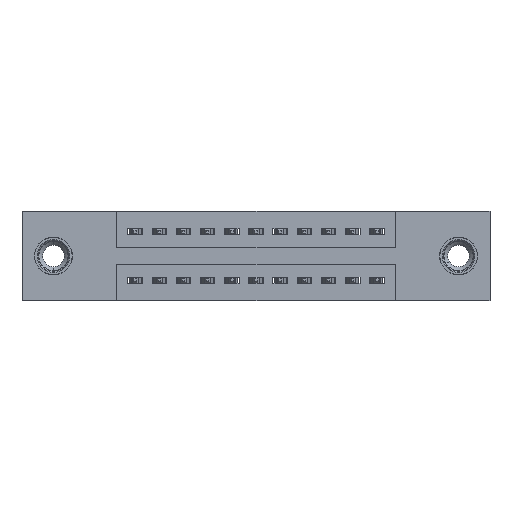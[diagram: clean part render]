
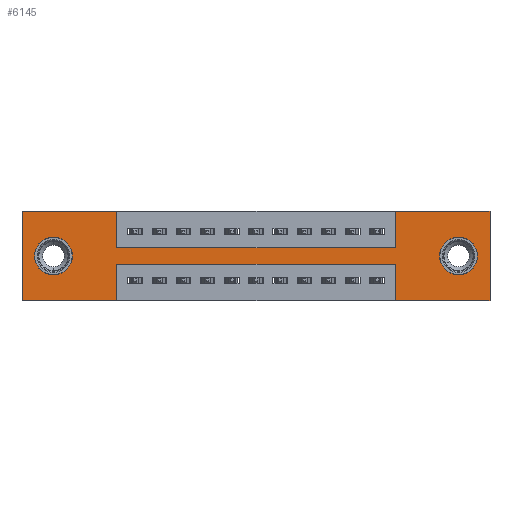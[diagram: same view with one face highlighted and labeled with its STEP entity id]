
A CAD part, front view. The second image highlights one B-rep face of the part: STEP entity #6145.
In plain terms, the highlighted planar face has unit normal (0, -1, 0).
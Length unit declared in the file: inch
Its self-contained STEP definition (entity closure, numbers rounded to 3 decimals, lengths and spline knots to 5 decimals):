
#20 = VERTEX_POINT ( 'NONE', #11122 ) ;
#23 = ORIENTED_EDGE ( 'NONE', *, *, #6052, .F. ) ;
#128 = ORIENTED_EDGE ( 'NONE', *, *, #2703, .F. ) ;
#165 = VERTEX_POINT ( 'NONE', #11045 ) ;
#206 = DIRECTION ( 'NONE',  ( 0., 0., 1. ) ) ;
#315 = EDGE_CURVE ( 'NONE', #11747, #10809, #11409, .T. ) ;
#462 = VECTOR ( 'NONE', #12750, 39.37008 ) ;
#887 = ORIENTED_EDGE ( 'NONE', *, *, #10371, .F. ) ;
#1019 = CARTESIAN_POINT ( 'NONE',  ( 1.935, 0., -0.37 ) ) ;
#1023 = VERTEX_POINT ( 'NONE', #4178 ) ;
#1107 = LINE ( 'NONE', #5156, #462 ) ;
#1495 = DIRECTION ( 'NONE',  ( -1., 0., 0. ) ) ;
#1529 = FACE_BOUND ( 'NONE', #7340, .T. ) ;
#1684 = VERTEX_POINT ( 'NONE', #13125 ) ;
#2119 = CARTESIAN_POINT ( 'NONE',  ( 0.3925, 0., -0.22 ) ) ;
#2204 = CARTESIAN_POINT ( 'NONE',  ( 0.13, 0., -0.185 ) ) ;
#2251 = CARTESIAN_POINT ( 'NONE',  ( 0.3925, 0., 0. ) ) ;
#2261 = LINE ( 'NONE', #10797, #5659 ) ;
#2303 = LINE ( 'NONE', #10645, #5187 ) ;
#2341 = AXIS2_PLACEMENT_3D ( 'NONE', #2204, #13065, #3444 ) ;
#2390 = VECTOR ( 'NONE', #1495, 39.37008 ) ;
#2434 = AXIS2_PLACEMENT_3D ( 'NONE', #13974, #2970, #11671 ) ;
#2435 = CARTESIAN_POINT ( 'NONE',  ( 0., 0., -0.37 ) ) ;
#2541 = EDGE_CURVE ( 'NONE', #13848, #13836, #4498, .T. ) ;
#2703 = EDGE_CURVE ( 'NONE', #4501, #13052, #9428, .T. ) ;
#2825 = CIRCLE ( 'NONE', #9827, 0.078 ) ;
#2970 = DIRECTION ( 'NONE',  ( 0., -1., 0. ) ) ;
#2999 = ORIENTED_EDGE ( 'NONE', *, *, #12667, .F. ) ;
#3106 = PLANE ( 'NONE',  #2434 ) ;
#3217 = VECTOR ( 'NONE', #10307, 39.37008 ) ;
#3347 = CARTESIAN_POINT ( 'NONE',  ( 0.13, 0., -0.107 ) ) ;
#3364 = CARTESIAN_POINT ( 'NONE',  ( 1.805, 0., -0.107 ) ) ;
#3444 = DIRECTION ( 'NONE',  ( 0., 0., 1. ) ) ;
#3503 = CARTESIAN_POINT ( 'NONE',  ( 0.3925, 0., -0.37 ) ) ;
#3883 = VECTOR ( 'NONE', #206, 39.37008 ) ;
#3990 = EDGE_CURVE ( 'NONE', #11073, #4501, #4802, .T. ) ;
#4178 = CARTESIAN_POINT ( 'NONE',  ( 1.935, 0., 0. ) ) ;
#4283 = VERTEX_POINT ( 'NONE', #6856 ) ;
#4307 = DIRECTION ( 'NONE',  ( 0., 1., 0. ) ) ;
#4315 = EDGE_CURVE ( 'NONE', #20, #11073, #8344, .T. ) ;
#4358 = CARTESIAN_POINT ( 'NONE',  ( 1.5425, 0., -0.37 ) ) ;
#4456 = VECTOR ( 'NONE', #9058, 39.37008 ) ;
#4498 = LINE ( 'NONE', #5763, #5514 ) ;
#4501 = VERTEX_POINT ( 'NONE', #6709 ) ;
#4526 = DIRECTION ( 'NONE',  ( 0., 0., -1. ) ) ;
#4534 = ORIENTED_EDGE ( 'NONE', *, *, #10204, .F. ) ;
#4769 = FACE_BOUND ( 'NONE', #14020, .T. ) ;
#4802 = LINE ( 'NONE', #2251, #5832 ) ;
#4848 = ORIENTED_EDGE ( 'NONE', *, *, #2541, .F. ) ;
#4930 = AXIS2_PLACEMENT_3D ( 'NONE', #10703, #9582, #11910 ) ;
#5156 = CARTESIAN_POINT ( 'NONE',  ( 1.935, 0., 0. ) ) ;
#5187 = VECTOR ( 'NONE', #11845, 39.37008 ) ;
#5188 = EDGE_CURVE ( 'NONE', #13836, #9325, #6814, .T. ) ;
#5395 = DIRECTION ( 'NONE',  ( -1., 0., 0. ) ) ;
#5418 = DIRECTION ( 'NONE',  ( 1., 0., 0. ) ) ;
#5426 = DIRECTION ( 'NONE',  ( 1., 0., 0. ) ) ;
#5514 = VECTOR ( 'NONE', #4526, 39.37008 ) ;
#5659 = VECTOR ( 'NONE', #5395, 39.37008 ) ;
#5763 = CARTESIAN_POINT ( 'NONE',  ( 0.3925, 0., -0.37 ) ) ;
#5832 = VECTOR ( 'NONE', #10734, 39.37008 ) ;
#5835 = ORIENTED_EDGE ( 'NONE', *, *, #8683, .F. ) ;
#5969 = ORIENTED_EDGE ( 'NONE', *, *, #11640, .F. ) ;
#6052 = EDGE_CURVE ( 'NONE', #8510, #1023, #6116, .T. ) ;
#6116 = LINE ( 'NONE', #9300, #3217 ) ;
#6145 = ADVANCED_FACE ( 'NONE', ( #4769, #1529, #9846 ), #3106, .T. ) ;
#6447 = CARTESIAN_POINT ( 'NONE',  ( 1.805, 0., -0.185 ) ) ;
#6582 = EDGE_CURVE ( 'NONE', #11406, #4283, #8632, .T. ) ;
#6709 = CARTESIAN_POINT ( 'NONE',  ( 0.3925, 0., -0.15 ) ) ;
#6809 = CARTESIAN_POINT ( 'NONE',  ( 0., 0., 0. ) ) ;
#6814 = LINE ( 'NONE', #2435, #12766 ) ;
#6856 = CARTESIAN_POINT ( 'NONE',  ( 0.13, 0., -0.263 ) ) ;
#6922 = DIRECTION ( 'NONE',  ( 0., 0., 1. ) ) ;
#6979 = CARTESIAN_POINT ( 'NONE',  ( 1.5425, 0., 0. ) ) ;
#7340 = EDGE_LOOP ( 'NONE', ( #11439, #11512 ) ) ;
#7367 = ORIENTED_EDGE ( 'NONE', *, *, #8702, .F. ) ;
#8245 = ORIENTED_EDGE ( 'NONE', *, *, #3990, .F. ) ;
#8321 = CARTESIAN_POINT ( 'NONE',  ( 0.3925, 0., -0.22 ) ) ;
#8344 = LINE ( 'NONE', #6809, #11421 ) ;
#8510 = VERTEX_POINT ( 'NONE', #6979 ) ;
#8632 = CIRCLE ( 'NONE', #10436, 0.078 ) ;
#8683 = EDGE_CURVE ( 'NONE', #1023, #13302, #1107, .T. ) ;
#8702 = EDGE_CURVE ( 'NONE', #9325, #20, #2303, .T. ) ;
#8724 = DIRECTION ( 'NONE',  ( 0., 0., -1. ) ) ;
#8741 = VECTOR ( 'NONE', #5418, 39.37008 ) ;
#8978 = CIRCLE ( 'NONE', #2341, 0.078 ) ;
#9058 = DIRECTION ( 'NONE',  ( 0., 0., 1. ) ) ;
#9300 = CARTESIAN_POINT ( 'NONE',  ( 0., 0., 0. ) ) ;
#9325 = VERTEX_POINT ( 'NONE', #10581 ) ;
#9428 = LINE ( 'NONE', #11932, #8741 ) ;
#9546 = LINE ( 'NONE', #11237, #4456 ) ;
#9582 = DIRECTION ( 'NONE',  ( 0., 1., 0. ) ) ;
#9827 = AXIS2_PLACEMENT_3D ( 'NONE', #6447, #4307, #8724 ) ;
#9846 = FACE_OUTER_BOUND ( 'NONE', #10379, .T. ) ;
#10076 = DIRECTION ( 'NONE',  ( -1., 0., 0. ) ) ;
#10204 = EDGE_CURVE ( 'NONE', #13302, #165, #2261, .T. ) ;
#10307 = DIRECTION ( 'NONE',  ( 1., 0., 0. ) ) ;
#10371 = EDGE_CURVE ( 'NONE', #13052, #8510, #9546, .T. ) ;
#10379 = EDGE_LOOP ( 'NONE', ( #4848, #5969, #2999, #4534, #5835, #23, #887, #128, #8245, #12338, #7367, #13858 ) ) ;
#10436 = AXIS2_PLACEMENT_3D ( 'NONE', #13606, #13417, #6922 ) ;
#10469 = CARTESIAN_POINT ( 'NONE',  ( 1.5425, 0., -0.15 ) ) ;
#10581 = CARTESIAN_POINT ( 'NONE',  ( 0., 0., -0.37 ) ) ;
#10645 = CARTESIAN_POINT ( 'NONE',  ( 0., 0., 0. ) ) ;
#10703 = CARTESIAN_POINT ( 'NONE',  ( 1.805, 0., -0.185 ) ) ;
#10734 = DIRECTION ( 'NONE',  ( 0., 0., -1. ) ) ;
#10797 = CARTESIAN_POINT ( 'NONE',  ( 0., 0., -0.37 ) ) ;
#10809 = VERTEX_POINT ( 'NONE', #3364 ) ;
#11045 = CARTESIAN_POINT ( 'NONE',  ( 1.5425, 0., -0.37 ) ) ;
#11073 = VERTEX_POINT ( 'NONE', #13703 ) ;
#11122 = CARTESIAN_POINT ( 'NONE',  ( 0., 0., 0. ) ) ;
#11237 = CARTESIAN_POINT ( 'NONE',  ( 1.5425, 0., 0. ) ) ;
#11406 = VERTEX_POINT ( 'NONE', #3347 ) ;
#11409 = CIRCLE ( 'NONE', #4930, 0.078 ) ;
#11421 = VECTOR ( 'NONE', #5426, 39.37008 ) ;
#11439 = ORIENTED_EDGE ( 'NONE', *, *, #6582, .T. ) ;
#11512 = ORIENTED_EDGE ( 'NONE', *, *, #13300, .T. ) ;
#11640 = EDGE_CURVE ( 'NONE', #1684, #13848, #13926, .T. ) ;
#11671 = DIRECTION ( 'NONE',  ( 0., 0., -1. ) ) ;
#11734 = ORIENTED_EDGE ( 'NONE', *, *, #13954, .T. ) ;
#11747 = VERTEX_POINT ( 'NONE', #12654 ) ;
#11845 = DIRECTION ( 'NONE',  ( 0., 0., 1. ) ) ;
#11910 = DIRECTION ( 'NONE',  ( 0., 0., -1. ) ) ;
#11932 = CARTESIAN_POINT ( 'NONE',  ( 0.3925, 0., -0.15 ) ) ;
#12222 = LINE ( 'NONE', #4358, #3883 ) ;
#12338 = ORIENTED_EDGE ( 'NONE', *, *, #4315, .F. ) ;
#12654 = CARTESIAN_POINT ( 'NONE',  ( 1.805, 0., -0.263 ) ) ;
#12667 = EDGE_CURVE ( 'NONE', #165, #1684, #12222, .T. ) ;
#12750 = DIRECTION ( 'NONE',  ( 0., 0., -1. ) ) ;
#12766 = VECTOR ( 'NONE', #10076, 39.37008 ) ;
#13016 = ORIENTED_EDGE ( 'NONE', *, *, #315, .T. ) ;
#13052 = VERTEX_POINT ( 'NONE', #10469 ) ;
#13065 = DIRECTION ( 'NONE',  ( 0., 1., 0. ) ) ;
#13125 = CARTESIAN_POINT ( 'NONE',  ( 1.5425, 0., -0.22 ) ) ;
#13300 = EDGE_CURVE ( 'NONE', #4283, #11406, #8978, .T. ) ;
#13302 = VERTEX_POINT ( 'NONE', #1019 ) ;
#13417 = DIRECTION ( 'NONE',  ( 0., 1., 0. ) ) ;
#13606 = CARTESIAN_POINT ( 'NONE',  ( 0.13, 0., -0.185 ) ) ;
#13703 = CARTESIAN_POINT ( 'NONE',  ( 0.3925, 0., 0. ) ) ;
#13836 = VERTEX_POINT ( 'NONE', #3503 ) ;
#13848 = VERTEX_POINT ( 'NONE', #2119 ) ;
#13858 = ORIENTED_EDGE ( 'NONE', *, *, #5188, .F. ) ;
#13926 = LINE ( 'NONE', #8321, #2390 ) ;
#13954 = EDGE_CURVE ( 'NONE', #10809, #11747, #2825, .T. ) ;
#13974 = CARTESIAN_POINT ( 'NONE',  ( 0., 0., -0.37 ) ) ;
#14020 = EDGE_LOOP ( 'NONE', ( #11734, #13016 ) ) ;
